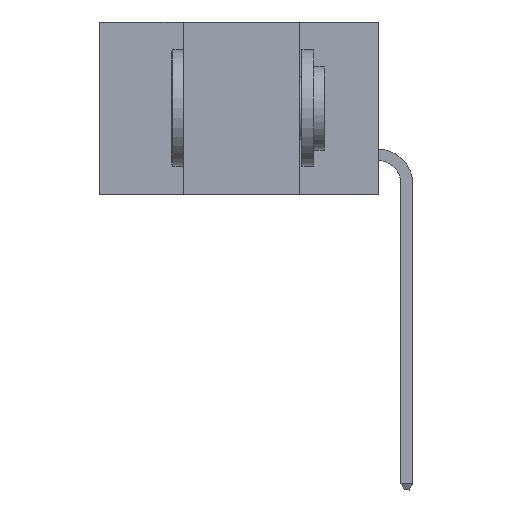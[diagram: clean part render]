
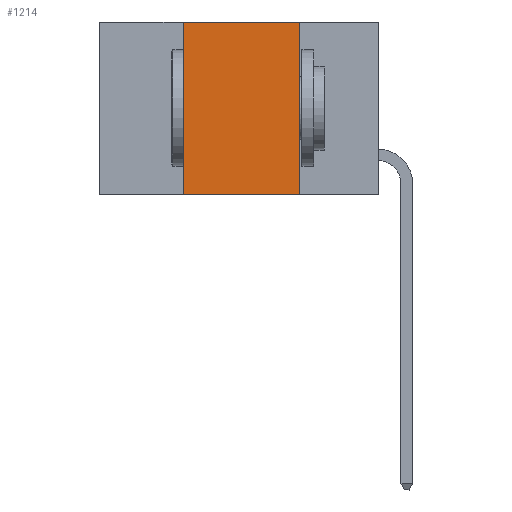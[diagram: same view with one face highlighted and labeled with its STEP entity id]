
A CAD part, left-side view. The second image highlights one B-rep face of the part: STEP entity #1214.
In plain terms, the highlighted planar face has unit normal (-1, 0, 0).
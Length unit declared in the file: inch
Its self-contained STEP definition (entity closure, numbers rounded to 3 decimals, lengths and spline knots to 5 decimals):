
#344 = VECTOR ( 'NONE', #18513, 39.37008 ) ;
#367 = FACE_OUTER_BOUND ( 'NONE', #11969, .T. ) ;
#1214 = ADVANCED_FACE ( 'NONE', ( #367 ), #5939, .F. ) ;
#1662 = EDGE_CURVE ( 'NONE', #10120, #11322, #6609, .T. ) ;
#2116 = CARTESIAN_POINT ( 'NONE',  ( 0., 0.42, -0.37 ) ) ;
#2341 = ORIENTED_EDGE ( 'NONE', *, *, #10208, .T. ) ;
#3250 = VECTOR ( 'NONE', #8538, 39.37008 ) ;
#3929 = ORIENTED_EDGE ( 'NONE', *, *, #1662, .F. ) ;
#5870 = ORIENTED_EDGE ( 'NONE', *, *, #9767, .F. ) ;
#5939 = PLANE ( 'NONE',  #18314 ) ;
#6319 = EDGE_CURVE ( 'NONE', #11322, #16883, #10045, .T. ) ;
#6447 = CARTESIAN_POINT ( 'NONE',  ( 0., 0.42, 0. ) ) ;
#6609 = LINE ( 'NONE', #24293, #344 ) ;
#7381 = CARTESIAN_POINT ( 'NONE',  ( 0., 0.17, 0. ) ) ;
#7955 = DIRECTION ( 'NONE',  ( 1., 0., 0. ) ) ;
#8538 = DIRECTION ( 'NONE',  ( 0., 0., 1. ) ) ;
#9643 = VERTEX_POINT ( 'NONE', #2116 ) ;
#9767 = EDGE_CURVE ( 'NONE', #9643, #10120, #12840, .T. ) ;
#9945 = CARTESIAN_POINT ( 'NONE',  ( 0., 0.6, 0. ) ) ;
#10045 = LINE ( 'NONE', #22978, #14529 ) ;
#10120 = VERTEX_POINT ( 'NONE', #6447 ) ;
#10208 = EDGE_CURVE ( 'NONE', #9643, #16883, #19702, .T. ) ;
#11158 = CARTESIAN_POINT ( 'NONE',  ( 0., 0.17, -0.37 ) ) ;
#11322 = VERTEX_POINT ( 'NONE', #7381 ) ;
#11969 = EDGE_LOOP ( 'NONE', ( #14366, #3929, #5870, #2341 ) ) ;
#12840 = LINE ( 'NONE', #16198, #3250 ) ;
#14366 = ORIENTED_EDGE ( 'NONE', *, *, #6319, .F. ) ;
#14529 = VECTOR ( 'NONE', #19300, 39.37008 ) ;
#16198 = CARTESIAN_POINT ( 'NONE',  ( 0., 0.42, 0. ) ) ;
#16883 = VERTEX_POINT ( 'NONE', #11158 ) ;
#18314 = AXIS2_PLACEMENT_3D ( 'NONE', #9945, #7955, #21387 ) ;
#18513 = DIRECTION ( 'NONE',  ( 0., -1., 0. ) ) ;
#18953 = DIRECTION ( 'NONE',  ( 0., -1., 0. ) ) ;
#19300 = DIRECTION ( 'NONE',  ( 0., 0., -1. ) ) ;
#19702 = LINE ( 'NONE', #24650, #22378 ) ;
#21387 = DIRECTION ( 'NONE',  ( 0., 0., -1. ) ) ;
#22378 = VECTOR ( 'NONE', #18953, 39.37008 ) ;
#22978 = CARTESIAN_POINT ( 'NONE',  ( 0., 0.17, 0. ) ) ;
#24293 = CARTESIAN_POINT ( 'NONE',  ( 0., 0.6, 0. ) ) ;
#24650 = CARTESIAN_POINT ( 'NONE',  ( 0., 0.6, -0.37 ) ) ;
